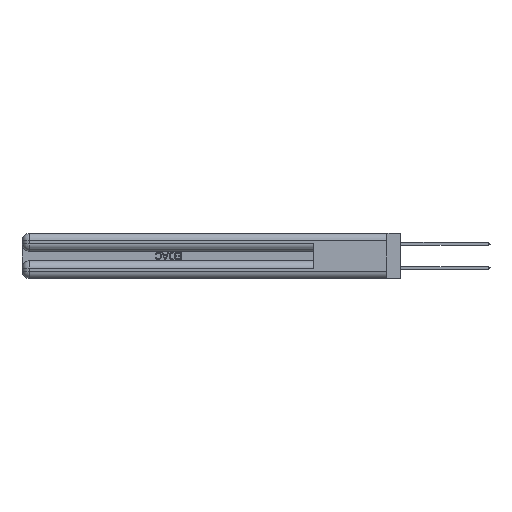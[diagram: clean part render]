
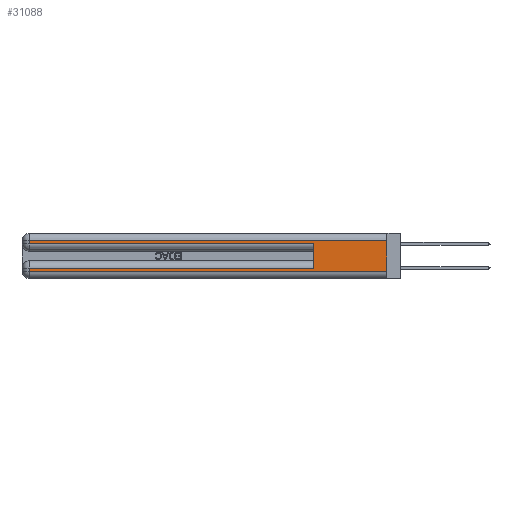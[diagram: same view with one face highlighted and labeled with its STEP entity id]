
A CAD part, left-side view. The second image highlights one B-rep face of the part: STEP entity #31088.
In plain terms, the highlighted planar face has unit normal (-1, 0, 0).
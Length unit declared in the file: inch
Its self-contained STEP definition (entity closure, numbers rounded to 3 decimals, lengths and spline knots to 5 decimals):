
#9 = DIRECTION ( 'NONE',  ( 0., 1., 0. ) ) ;
#83 = CARTESIAN_POINT ( 'NONE',  ( 0., 2.94, 0.285 ) ) ;
#618 = EDGE_CURVE ( 'NONE', #1084, #14518, #50500, .T. ) ;
#1084 = VERTEX_POINT ( 'NONE', #46414 ) ;
#1152 = CARTESIAN_POINT ( 'NONE',  ( 0., 2.94, 0.37 ) ) ;
#5136 = VECTOR ( 'NONE', #16212, 39.37008 ) ;
#5555 = DIRECTION ( 'NONE',  ( 0., 0., -1. ) ) ;
#6513 = LINE ( 'NONE', #54637, #5136 ) ;
#6756 = DIRECTION ( 'NONE',  ( 0., 0., -1. ) ) ;
#7649 = VECTOR ( 'NONE', #14825, 39.37008 ) ;
#7813 = DIRECTION ( 'NONE',  ( 0., -1., 0. ) ) ;
#8353 = VERTEX_POINT ( 'NONE', #48405 ) ;
#9301 = CARTESIAN_POINT ( 'NONE',  ( 0., 2.94, 0.37 ) ) ;
#10496 = CARTESIAN_POINT ( 'NONE',  ( 0., 0., 0.37 ) ) ;
#11134 = ORIENTED_EDGE ( 'NONE', *, *, #41710, .F. ) ;
#12432 = VERTEX_POINT ( 'NONE', #83 ) ;
#13181 = EDGE_CURVE ( 'NONE', #16840, #47866, #48285, .T. ) ;
#13624 = DIRECTION ( 'NONE',  ( 0., 0., -1. ) ) ;
#13816 = EDGE_CURVE ( 'NONE', #14518, #12432, #52911, .T. ) ;
#14000 = CARTESIAN_POINT ( 'NONE',  ( 0., 0.6, 0.145 ) ) ;
#14510 = EDGE_CURVE ( 'NONE', #34289, #16840, #6513, .T. ) ;
#14518 = VERTEX_POINT ( 'NONE', #54823 ) ;
#14825 = DIRECTION ( 'NONE',  ( 0., 0., -1. ) ) ;
#14891 = VERTEX_POINT ( 'NONE', #36267 ) ;
#15658 = CARTESIAN_POINT ( 'NONE',  ( 0., 0.6, 0.085 ) ) ;
#16212 = DIRECTION ( 'NONE',  ( 0., 1., 0. ) ) ;
#16257 = VECTOR ( 'NONE', #9, 39.37008 ) ;
#16840 = VERTEX_POINT ( 'NONE', #44319 ) ;
#17195 = CARTESIAN_POINT ( 'NONE',  ( 0., 0., 0.31 ) ) ;
#17594 = EDGE_CURVE ( 'NONE', #47866, #8353, #47888, .T. ) ;
#18271 = DIRECTION ( 'NONE',  ( 0., 0., 1. ) ) ;
#20725 = CARTESIAN_POINT ( 'NONE',  ( 0., 0., 0.06 ) ) ;
#20737 = CARTESIAN_POINT ( 'NONE',  ( 0., 0., 0.285 ) ) ;
#23622 = CARTESIAN_POINT ( 'NONE',  ( 0., 0., 0.37 ) ) ;
#24350 = FACE_OUTER_BOUND ( 'NONE', #55390, .T. ) ;
#25049 = VECTOR ( 'NONE', #7813, 39.37008 ) ;
#25050 = EDGE_CURVE ( 'NONE', #1084, #8353, #44573, .T. ) ;
#25058 = DIRECTION ( 'NONE',  ( 0., -1., 0. ) ) ;
#25958 = VECTOR ( 'NONE', #25058, 39.37008 ) ;
#28143 = PLANE ( 'NONE',  #40246 ) ;
#28329 = LINE ( 'NONE', #14000, #49831 ) ;
#31088 = ADVANCED_FACE ( 'NONE', ( #24350 ), #28143, .F. ) ;
#32508 = DIRECTION ( 'NONE',  ( 1., 0., 0. ) ) ;
#34125 = ORIENTED_EDGE ( 'NONE', *, *, #39116, .T. ) ;
#34289 = VERTEX_POINT ( 'NONE', #15658 ) ;
#36267 = CARTESIAN_POINT ( 'NONE',  ( 0., 0.6, 0.285 ) ) ;
#36895 = VECTOR ( 'NONE', #5555, 39.37008 ) ;
#37520 = ORIENTED_EDGE ( 'NONE', *, *, #25050, .F. ) ;
#38777 = LINE ( 'NONE', #20737, #25958 ) ;
#39116 = EDGE_CURVE ( 'NONE', #12432, #14891, #38777, .T. ) ;
#40246 = AXIS2_PLACEMENT_3D ( 'NONE', #23622, #32508, #6756 ) ;
#41536 = VECTOR ( 'NONE', #13624, 39.37008 ) ;
#41710 = EDGE_CURVE ( 'NONE', #34289, #14891, #28329, .T. ) ;
#42092 = ORIENTED_EDGE ( 'NONE', *, *, #14510, .T. ) ;
#44319 = CARTESIAN_POINT ( 'NONE',  ( 0., 2.94, 0.085 ) ) ;
#44573 = LINE ( 'NONE', #10496, #7649 ) ;
#44982 = ORIENTED_EDGE ( 'NONE', *, *, #13816, .T. ) ;
#46414 = CARTESIAN_POINT ( 'NONE',  ( 0., 0., 0.31 ) ) ;
#47866 = VERTEX_POINT ( 'NONE', #50986 ) ;
#47888 = LINE ( 'NONE', #20725, #25049 ) ;
#47938 = ORIENTED_EDGE ( 'NONE', *, *, #13181, .T. ) ;
#48285 = LINE ( 'NONE', #1152, #36895 ) ;
#48405 = CARTESIAN_POINT ( 'NONE',  ( 0., 0., 0.06 ) ) ;
#48442 = ORIENTED_EDGE ( 'NONE', *, *, #618, .T. ) ;
#49831 = VECTOR ( 'NONE', #18271, 39.37008 ) ;
#50500 = LINE ( 'NONE', #17195, #16257 ) ;
#50986 = CARTESIAN_POINT ( 'NONE',  ( 0., 2.94, 0.06 ) ) ;
#52911 = LINE ( 'NONE', #9301, #41536 ) ;
#53223 = ORIENTED_EDGE ( 'NONE', *, *, #17594, .T. ) ;
#54637 = CARTESIAN_POINT ( 'NONE',  ( 0., 0., 0.085 ) ) ;
#54823 = CARTESIAN_POINT ( 'NONE',  ( 0., 2.94, 0.31 ) ) ;
#55390 = EDGE_LOOP ( 'NONE', ( #37520, #48442, #44982, #34125, #11134, #42092, #47938, #53223 ) ) ;
